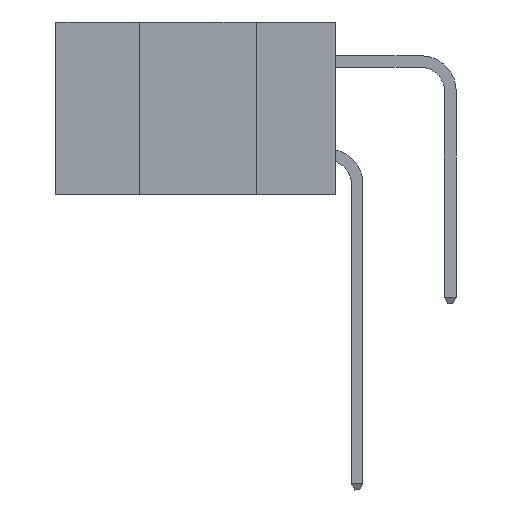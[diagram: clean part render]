
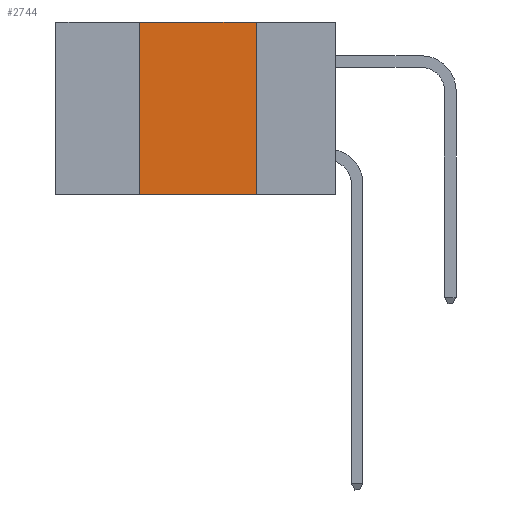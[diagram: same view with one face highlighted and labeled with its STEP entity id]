
A CAD part, left-side view. The second image highlights one B-rep face of the part: STEP entity #2744.
In plain terms, the highlighted planar face has unit normal (-1, 0, 0).
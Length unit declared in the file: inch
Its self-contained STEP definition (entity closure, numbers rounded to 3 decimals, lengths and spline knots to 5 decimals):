
#1649 = VERTEX_POINT ( 'NONE', #15996 ) ;
#1879 = VECTOR ( 'NONE', #8017, 39.37008 ) ;
#2484 = VERTEX_POINT ( 'NONE', #5002 ) ;
#2595 = DIRECTION ( 'NONE',  ( 0., -1., 0. ) ) ;
#2744 = ADVANCED_FACE ( 'NONE', ( #5280 ), #17842, .F. ) ;
#3457 = VERTEX_POINT ( 'NONE', #8235 ) ;
#3750 = LINE ( 'NONE', #8586, #24656 ) ;
#5002 = CARTESIAN_POINT ( 'NONE',  ( 0., 0.42, 0. ) ) ;
#5280 = FACE_OUTER_BOUND ( 'NONE', #17151, .T. ) ;
#5962 = CARTESIAN_POINT ( 'NONE',  ( 0., 0.42, 0. ) ) ;
#6949 = ORIENTED_EDGE ( 'NONE', *, *, #14645, .T. ) ;
#7422 = LINE ( 'NONE', #5962, #1879 ) ;
#8017 = DIRECTION ( 'NONE',  ( 0., 0., 1. ) ) ;
#8235 = CARTESIAN_POINT ( 'NONE',  ( 0., 0.42, -0.37 ) ) ;
#8586 = CARTESIAN_POINT ( 'NONE',  ( 0., 0.6, 0. ) ) ;
#9534 = VECTOR ( 'NONE', #11404, 39.37008 ) ;
#9562 = ORIENTED_EDGE ( 'NONE', *, *, #22889, .F. ) ;
#10695 = DIRECTION ( 'NONE',  ( 0., -1., 0. ) ) ;
#11404 = DIRECTION ( 'NONE',  ( 0., 0., -1. ) ) ;
#11732 = CARTESIAN_POINT ( 'NONE',  ( 0., 0.6, 0. ) ) ;
#13170 = EDGE_CURVE ( 'NONE', #3457, #2484, #7422, .T. ) ;
#14645 = EDGE_CURVE ( 'NONE', #3457, #23631, #19890, .T. ) ;
#15032 = LINE ( 'NONE', #15532, #9534 ) ;
#15040 = CARTESIAN_POINT ( 'NONE',  ( 0., 0.6, -0.37 ) ) ;
#15532 = CARTESIAN_POINT ( 'NONE',  ( 0., 0.17, 0. ) ) ;
#15701 = ORIENTED_EDGE ( 'NONE', *, *, #13170, .F. ) ;
#15840 = CARTESIAN_POINT ( 'NONE',  ( 0., 0.17, -0.37 ) ) ;
#15996 = CARTESIAN_POINT ( 'NONE',  ( 0., 0.17, 0. ) ) ;
#17151 = EDGE_LOOP ( 'NONE', ( #9562, #24903, #15701, #6949 ) ) ;
#17532 = EDGE_CURVE ( 'NONE', #2484, #1649, #3750, .T. ) ;
#17842 = PLANE ( 'NONE',  #20725 ) ;
#19890 = LINE ( 'NONE', #15040, #25109 ) ;
#20725 = AXIS2_PLACEMENT_3D ( 'NONE', #11732, #26036, #21283 ) ;
#21283 = DIRECTION ( 'NONE',  ( 0., 0., -1. ) ) ;
#22889 = EDGE_CURVE ( 'NONE', #1649, #23631, #15032, .T. ) ;
#23631 = VERTEX_POINT ( 'NONE', #15840 ) ;
#24656 = VECTOR ( 'NONE', #10695, 39.37008 ) ;
#24903 = ORIENTED_EDGE ( 'NONE', *, *, #17532, .F. ) ;
#25109 = VECTOR ( 'NONE', #2595, 39.37008 ) ;
#26036 = DIRECTION ( 'NONE',  ( 1., 0., 0. ) ) ;
